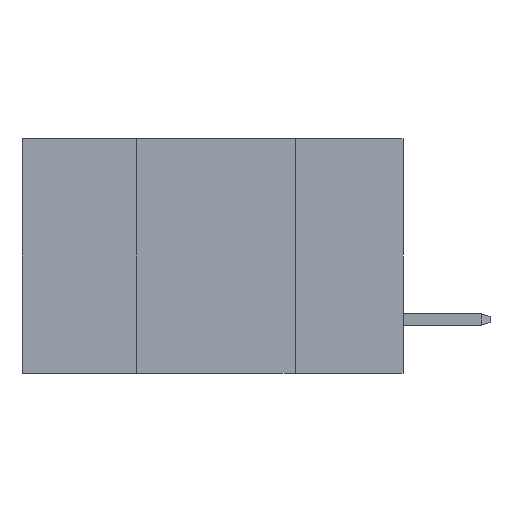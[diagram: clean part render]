
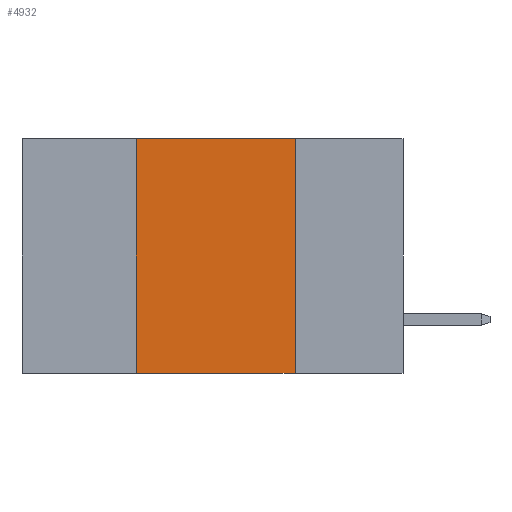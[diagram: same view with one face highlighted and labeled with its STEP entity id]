
A CAD part, left-side view. The second image highlights one B-rep face of the part: STEP entity #4932.
In plain terms, the highlighted planar face has unit normal (-1, 0, 0).
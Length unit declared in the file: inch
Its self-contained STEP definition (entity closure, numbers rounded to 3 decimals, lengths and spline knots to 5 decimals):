
#10 = AXIS2_PLACEMENT_3D ( 'NONE', #4815, #1441, #3486 ) ;
#85 = VERTEX_POINT ( 'NONE', #2272 ) ;
#216 = LINE ( 'NONE', #3524, #7071 ) ;
#851 = FACE_OUTER_BOUND ( 'NONE', #8744, .T. ) ;
#1129 = LINE ( 'NONE', #1725, #1374 ) ;
#1374 = VECTOR ( 'NONE', #1761, 39.37008 ) ;
#1441 = DIRECTION ( 'NONE',  ( 1., 0., 0. ) ) ;
#1725 = CARTESIAN_POINT ( 'NONE',  ( 0., 0.6, 0. ) ) ;
#1761 = DIRECTION ( 'NONE',  ( 0., -1., 0. ) ) ;
#2040 = ORIENTED_EDGE ( 'NONE', *, *, #7611, .T. ) ;
#2272 = CARTESIAN_POINT ( 'NONE',  ( 0., 0.42, -0.37 ) ) ;
#2855 = VERTEX_POINT ( 'NONE', #5190 ) ;
#3486 = DIRECTION ( 'NONE',  ( 0., 0., -1. ) ) ;
#3524 = CARTESIAN_POINT ( 'NONE',  ( 0., 0.6, -0.37 ) ) ;
#4157 = ORIENTED_EDGE ( 'NONE', *, *, #7215, .F. ) ;
#4278 = PLANE ( 'NONE',  #10 ) ;
#4397 = VECTOR ( 'NONE', #8934, 39.37008 ) ;
#4422 = DIRECTION ( 'NONE',  ( 0., 0., 1. ) ) ;
#4815 = CARTESIAN_POINT ( 'NONE',  ( 0., 0.6, 0. ) ) ;
#4932 = ADVANCED_FACE ( 'NONE', ( #851 ), #4278, .F. ) ;
#5157 = VERTEX_POINT ( 'NONE', #6922 ) ;
#5190 = CARTESIAN_POINT ( 'NONE',  ( 0., 0.17, -0.37 ) ) ;
#5554 = LINE ( 'NONE', #8463, #8193 ) ;
#5745 = ORIENTED_EDGE ( 'NONE', *, *, #7993, .F. ) ;
#6922 = CARTESIAN_POINT ( 'NONE',  ( 0., 0.42, 0. ) ) ;
#7071 = VECTOR ( 'NONE', #8484, 39.37008 ) ;
#7215 = EDGE_CURVE ( 'NONE', #7621, #2855, #8209, .T. ) ;
#7529 = CARTESIAN_POINT ( 'NONE',  ( 0., 0.17, 0. ) ) ;
#7611 = EDGE_CURVE ( 'NONE', #85, #2855, #216, .T. ) ;
#7621 = VERTEX_POINT ( 'NONE', #7739 ) ;
#7739 = CARTESIAN_POINT ( 'NONE',  ( 0., 0.17, 0. ) ) ;
#7757 = EDGE_CURVE ( 'NONE', #5157, #7621, #1129, .T. ) ;
#7993 = EDGE_CURVE ( 'NONE', #85, #5157, #5554, .T. ) ;
#8193 = VECTOR ( 'NONE', #4422, 39.37008 ) ;
#8209 = LINE ( 'NONE', #7529, #4397 ) ;
#8463 = CARTESIAN_POINT ( 'NONE',  ( 0., 0.42, 0. ) ) ;
#8484 = DIRECTION ( 'NONE',  ( 0., -1., 0. ) ) ;
#8744 = EDGE_LOOP ( 'NONE', ( #4157, #8904, #5745, #2040 ) ) ;
#8904 = ORIENTED_EDGE ( 'NONE', *, *, #7757, .F. ) ;
#8934 = DIRECTION ( 'NONE',  ( 0., 0., -1. ) ) ;
